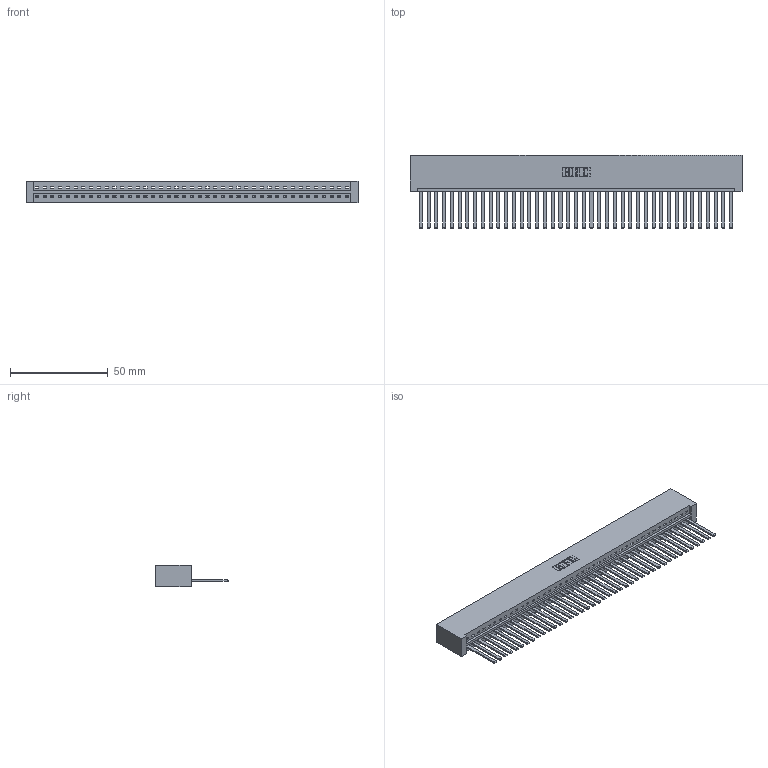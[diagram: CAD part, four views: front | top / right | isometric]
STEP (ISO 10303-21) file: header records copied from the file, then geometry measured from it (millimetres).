
FILE_DESCRIPTION (( 'STEP AP203' ), '1' );
FILE_NAME ('336-041-541-601.STEP', '2020-08-07T23:25:35', ( '' ), ( '' ), 'SwSTEP 2.0', 'SolidWorks 2020', '' );
FILE_SCHEMA (( 'CONFIG_CONTROL_DESIGN' ));
Length unit declared in the file: inch
Products named in the file (3): 336 Part_Lugless; 336-041-541-601; 336-290-001_336-290-541
Assembly tree (42 placements, depth 2):
  336-041-541-601
    336 Part_Lugless
    336-290-001_336-290-541  x41
Bounding box: 169.57 x 37.34 x 11.1 mm (x, y, z)
Volume: 26213.6 mm3; surface area: 28554.1 mm2
Topology: 42 solids, 42 shells, 2156 faces, 6601 edges, 4372 vertices
Faces by surface type: plane 1460, cylinder 696
Entity records: 30048 total; most frequent: CARTESIAN_POINT 5324, ORIENTED_EDGE 5202, DIRECTION 4379, EDGE_CURVE 2601, VECTOR 2477, LINE 2477, VERTEX_POINT 1732, AXIS2_PLACEMENT_3D 951
